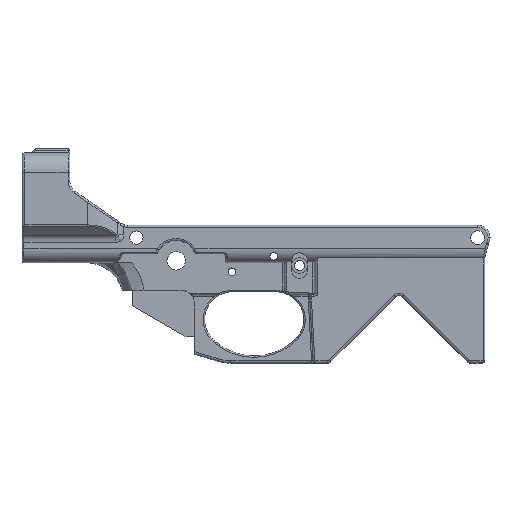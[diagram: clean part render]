
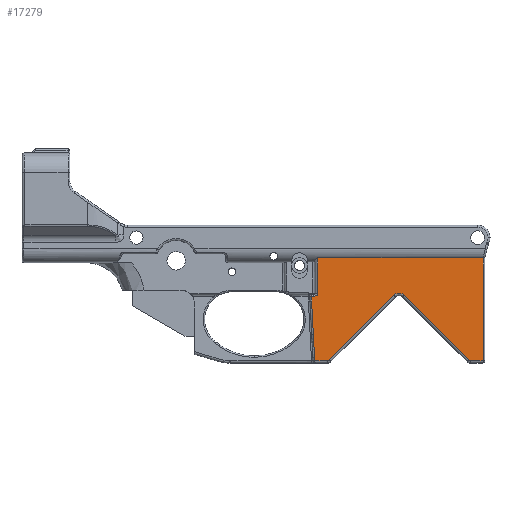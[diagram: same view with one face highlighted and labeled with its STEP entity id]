
A CAD part, front view. The second image highlights one B-rep face of the part: STEP entity #17279.
In plain terms, the highlighted planar face has unit normal (0, -1, 0).
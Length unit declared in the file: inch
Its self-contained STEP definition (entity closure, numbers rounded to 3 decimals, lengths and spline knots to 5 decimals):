
#18 = CARTESIAN_POINT ( 'NONE',  ( 1.54798, -1.41927, -0.98747 ) ) ;
#257 = ORIENTED_EDGE ( 'NONE', *, *, #27352, .T. ) ;
#749 = CARTESIAN_POINT ( 'NONE',  ( 2.19048, -1.41927, -0.94157 ) ) ;
#767 = VERTEX_POINT ( 'NONE', #32635 ) ;
#848 = ORIENTED_EDGE ( 'NONE', *, *, #12026, .F. ) ;
#1169 = LINE ( 'NONE', #11966, #15663 ) ;
#1539 = CARTESIAN_POINT ( 'NONE',  ( 3.82453, -1.41927, -1.07605 ) ) ;
#1572 = VERTEX_POINT ( 'NONE', #32628 ) ;
#2049 = CIRCLE ( 'NONE', #37120, 0.05 ) ;
#2088 = ORIENTED_EDGE ( 'NONE', *, *, #28652, .T. ) ;
#2500 = DIRECTION ( 'NONE',  ( 0., 0., -1. ) ) ;
#2837 = VERTEX_POINT ( 'NONE', #27662 ) ;
#2845 = CIRCLE ( 'NONE', #31849, 0.05 ) ;
#3069 = ORIENTED_EDGE ( 'NONE', *, *, #3202, .T. ) ;
#3202 = EDGE_CURVE ( 'NONE', #27405, #1572, #1169, .T. ) ;
#3377 = LINE ( 'NONE', #18, #33172 ) ;
#4308 = CARTESIAN_POINT ( 'NONE',  ( 2.38092, -1.41927, -2.23681 ) ) ;
#4324 = ORIENTED_EDGE ( 'NONE', *, *, #27732, .T. ) ;
#4481 = DIRECTION ( 'NONE',  ( 1., 0., 0. ) ) ;
#4578 = CARTESIAN_POINT ( 'NONE',  ( 5.26814, -1.41927, -2.28681 ) ) ;
#4754 = CARTESIAN_POINT ( 'NONE',  ( 2.19048, -1.41927, -0.93551 ) ) ;
#4830 = EDGE_CURVE ( 'NONE', #30923, #2837, #3377, .T. ) ;
#4949 = DIRECTION ( 'NONE',  ( 1., 0., 0. ) ) ;
#5137 = VECTOR ( 'NONE', #21559, 39.37008 ) ;
#5228 = VECTOR ( 'NONE', #15095, 39.37008 ) ;
#5253 = CARTESIAN_POINT ( 'NONE',  ( 2.19048, -1.41927, -0.21677 ) ) ;
#6002 = EDGE_CURVE ( 'NONE', #31784, #29235, #21087, .T. ) ;
#6436 = CARTESIAN_POINT ( 'NONE',  ( 2.06298, -1.41927, -0.72309 ) ) ;
#6916 = ORIENTED_EDGE ( 'NONE', *, *, #4830, .T. ) ;
#7227 = DIRECTION ( 'NONE',  ( 1., 0., 0. ) ) ;
#7439 = EDGE_CURVE ( 'NONE', #767, #20061, #28205, .T. ) ;
#7492 = AXIS2_PLACEMENT_3D ( 'NONE', #37116, #19798, #2500 ) ;
#7623 = CARTESIAN_POINT ( 'NONE',  ( 3.71847, -1.41927, -0.96998 ) ) ;
#7627 = ORIENTED_EDGE ( 'NONE', *, *, #6002, .T. ) ;
#7727 = VERTEX_POINT ( 'NONE', #19608 ) ;
#7883 = DIRECTION ( 'NONE',  ( 0.707, 0., -0.707 ) ) ;
#7986 = CARTESIAN_POINT ( 'NONE',  ( 5.52051, -1.41927, -2.28681 ) ) ;
#8481 = VECTOR ( 'NONE', #28549, 39.37008 ) ;
#9326 = DIRECTION ( 'NONE',  ( 0., 0., -1. ) ) ;
#9418 = EDGE_CURVE ( 'NONE', #32424, #15975, #2049, .T. ) ;
#9503 = CARTESIAN_POINT ( 'NONE',  ( 2.41628, -1.41927, -2.27217 ) ) ;
#9925 = CARTESIAN_POINT ( 'NONE',  ( 5.26814, -1.41927, -2.23681 ) ) ;
#9995 = LINE ( 'NONE', #22363, #16723 ) ;
#10956 = CARTESIAN_POINT ( 'NONE',  ( 2.19048, -1.41927, -0.92747 ) ) ;
#11043 = EDGE_CURVE ( 'NONE', #7727, #12313, #2845, .T. ) ;
#11382 = VECTOR ( 'NONE', #23870, 39.37008 ) ;
#11424 = ORIENTED_EDGE ( 'NONE', *, *, #23147, .F. ) ;
#11966 = CARTESIAN_POINT ( 'NONE',  ( 5.52051, -1.41927, -17.50299 ) ) ;
#12026 = EDGE_CURVE ( 'NONE', #30349, #767, #12285, .T. ) ;
#12155 = CARTESIAN_POINT ( 'NONE',  ( 2.11048, -1.41927, -0.98747 ) ) ;
#12283 = CARTESIAN_POINT ( 'NONE',  ( 2.14794, -1.41927, -0.9813 ) ) ;
#12285 = LINE ( 'NONE', #20980, #11382 ) ;
#12313 = VERTEX_POINT ( 'NONE', #4578 ) ;
#12831 = DIRECTION ( 'NONE',  ( 1., 0., 0. ) ) ;
#13588 = DIRECTION ( 'NONE',  ( 0., 0., -1. ) ) ;
#14510 = LINE ( 'NONE', #6436, #28923 ) ;
#14650 = CARTESIAN_POINT ( 'NONE',  ( 2.38092, -1.41927, -2.28681 ) ) ;
#15095 = DIRECTION ( 'NONE',  ( -0.052, 0., 0.999 ) ) ;
#15186 = CARTESIAN_POINT ( 'NONE',  ( 2.16989, -1.41927, -0.96975 ) ) ;
#15663 = VECTOR ( 'NONE', #17753, 39.37008 ) ;
#15975 = VERTEX_POINT ( 'NONE', #9503 ) ;
#16141 = LINE ( 'NONE', #22769, #8481 ) ;
#16723 = VECTOR ( 'NONE', #7883, 39.37008 ) ;
#16734 = ORIENTED_EDGE ( 'NONE', *, *, #9418, .T. ) ;
#16827 = VECTOR ( 'NONE', #32926, 39.37008 ) ;
#17056 = VERTEX_POINT ( 'NONE', #18942 ) ;
#17071 = VERTEX_POINT ( 'NONE', #7623 ) ;
#17279 = ADVANCED_FACE ( 'NONE', ( #17798 ), #22578, .T. ) ;
#17389 = ORIENTED_EDGE ( 'NONE', *, *, #21094, .T. ) ;
#17722 = LINE ( 'NONE', #24226, #16827 ) ;
#17753 = DIRECTION ( 'NONE',  ( 0., 0., 1. ) ) ;
#17779 = LINE ( 'NONE', #36757, #33135 ) ;
#17798 = FACE_OUTER_BOUND ( 'NONE', #20186, .T. ) ;
#17859 = CARTESIAN_POINT ( 'NONE',  ( 2.13832, -1.41927, -2.52309 ) ) ;
#18060 = CARTESIAN_POINT ( 'NONE',  ( 2.1863, -1.41927, -0.95037 ) ) ;
#18512 = AXIS2_PLACEMENT_3D ( 'NONE', #1539, #21761, #4481 ) ;
#18655 = CARTESIAN_POINT ( 'NONE',  ( 2.96195, -1.41927, -0.21677 ) ) ;
#18942 = CARTESIAN_POINT ( 'NONE',  ( 3.9306, -1.41927, -0.96998 ) ) ;
#18945 = CARTESIAN_POINT ( 'NONE',  ( 2.12594, -1.41927, -2.28681 ) ) ;
#19608 = CARTESIAN_POINT ( 'NONE',  ( 5.23278, -1.41927, -2.27217 ) ) ;
#19741 = ORIENTED_EDGE ( 'NONE', *, *, #33486, .T. ) ;
#19798 = DIRECTION ( 'NONE',  ( 0., -1., 0. ) ) ;
#20061 = VERTEX_POINT ( 'NONE', #20624 ) ;
#20186 = EDGE_LOOP ( 'NONE', ( #4324, #7627, #11424, #6916, #22814, #32051, #848, #31226, #16734, #19741, #2088, #17389, #20416, #257, #3069 ) ) ;
#20238 = DIRECTION ( 'NONE',  ( -1., 0., 0. ) ) ;
#20416 = ORIENTED_EDGE ( 'NONE', *, *, #11043, .T. ) ;
#20624 = CARTESIAN_POINT ( 'NONE',  ( 2.06298, -1.41927, -1.08552 ) ) ;
#20834 = CARTESIAN_POINT ( 'NONE',  ( 2.12128, -1.41927, -0.98747 ) ) ;
#20970 = CARTESIAN_POINT ( 'NONE',  ( 2.19048, -1.41927, -0.92747 ) ) ;
#20980 = CARTESIAN_POINT ( 'NONE',  ( 2.1621, -1.41927, -2.97691 ) ) ;
#21087 = LINE ( 'NONE', #4754, #35559 ) ;
#21094 = EDGE_CURVE ( 'NONE', #17056, #7727, #9995, .T. ) ;
#21559 = DIRECTION ( 'NONE',  ( -1., 0., 0. ) ) ;
#21761 = DIRECTION ( 'NONE',  ( 0., 1., 0. ) ) ;
#22363 = CARTESIAN_POINT ( 'NONE',  ( 5.23278, -1.41927, -2.27217 ) ) ;
#22578 = PLANE ( 'NONE',  #7492 ) ;
#22769 = CARTESIAN_POINT ( 'NONE',  ( 3.71847, -1.41927, -0.96998 ) ) ;
#22814 = ORIENTED_EDGE ( 'NONE', *, *, #28900, .T. ) ;
#23147 = EDGE_CURVE ( 'NONE', #30923, #29235, #23691, .T. ) ;
#23691 = B_SPLINE_CURVE_WITH_KNOTS ( 'NONE', 3,
 ( #12155, #20834, #29530, #12283, #32421, #15186, #35370, #18060, #749, #20970 ),
 .UNSPECIFIED., .F., .F.,
 ( 4, 2, 2, 2, 4 ),
 ( 0., 0.25, 0.5, 0.75, 1. ),
 .UNSPECIFIED. ) ;
#23870 = DIRECTION ( 'NONE',  ( -0.052, 0., 0.999 ) ) ;
#24226 = CARTESIAN_POINT ( 'NONE',  ( 1.54798, -1.41927, -2.28681 ) ) ;
#24455 = DIRECTION ( 'NONE',  ( 0., -1., 0. ) ) ;
#27215 = LINE ( 'NONE', #18655, #5137 ) ;
#27352 = EDGE_CURVE ( 'NONE', #12313, #27405, #17779, .T. ) ;
#27405 = VERTEX_POINT ( 'NONE', #7986 ) ;
#27662 = CARTESIAN_POINT ( 'NONE',  ( 2.06298, -1.41927, -0.98747 ) ) ;
#27732 = EDGE_CURVE ( 'NONE', #1572, #31784, #27215, .T. ) ;
#28205 = LINE ( 'NONE', #17859, #5228 ) ;
#28470 = CIRCLE ( 'NONE', #18512, 0.15 ) ;
#28549 = DIRECTION ( 'NONE',  ( 0.707, 0., 0.707 ) ) ;
#28652 = EDGE_CURVE ( 'NONE', #17071, #17056, #28470, .T. ) ;
#28900 = EDGE_CURVE ( 'NONE', #2837, #20061, #14510, .T. ) ;
#28923 = VECTOR ( 'NONE', #9326, 39.37008 ) ;
#29235 = VERTEX_POINT ( 'NONE', #10956 ) ;
#29530 = CARTESIAN_POINT ( 'NONE',  ( 2.13069, -1.41927, -0.98595 ) ) ;
#30052 = DIRECTION ( 'NONE',  ( 0., -1., 0. ) ) ;
#30349 = VERTEX_POINT ( 'NONE', #18945 ) ;
#30923 = VERTEX_POINT ( 'NONE', #32496 ) ;
#31226 = ORIENTED_EDGE ( 'NONE', *, *, #36966, .T. ) ;
#31784 = VERTEX_POINT ( 'NONE', #5253 ) ;
#31849 = AXIS2_PLACEMENT_3D ( 'NONE', #9925, #30052, #12831 ) ;
#32051 = ORIENTED_EDGE ( 'NONE', *, *, #7439, .F. ) ;
#32421 = CARTESIAN_POINT ( 'NONE',  ( 2.15577, -1.41927, -0.97813 ) ) ;
#32424 = VERTEX_POINT ( 'NONE', #14650 ) ;
#32496 = CARTESIAN_POINT ( 'NONE',  ( 2.11048, -1.41927, -0.98747 ) ) ;
#32628 = CARTESIAN_POINT ( 'NONE',  ( 5.52051, -1.41927, -0.21677 ) ) ;
#32635 = CARTESIAN_POINT ( 'NONE',  ( 2.0982, -1.41927, -1.75761 ) ) ;
#32926 = DIRECTION ( 'NONE',  ( 1., 0., 0. ) ) ;
#33135 = VECTOR ( 'NONE', #4949, 39.37008 ) ;
#33172 = VECTOR ( 'NONE', #20238, 39.37008 ) ;
#33486 = EDGE_CURVE ( 'NONE', #15975, #17071, #16141, .T. ) ;
#35370 = CARTESIAN_POINT ( 'NONE',  ( 2.17622, -1.41927, -0.96456 ) ) ;
#35559 = VECTOR ( 'NONE', #13588, 39.37008 ) ;
#36757 = CARTESIAN_POINT ( 'NONE',  ( 1.54798, -1.41927, -2.28681 ) ) ;
#36966 = EDGE_CURVE ( 'NONE', #30349, #32424, #17722, .T. ) ;
#37116 = CARTESIAN_POINT ( 'NONE',  ( 1.54798, -1.41927, 0.44253 ) ) ;
#37120 = AXIS2_PLACEMENT_3D ( 'NONE', #4308, #24455, #7227 ) ;
